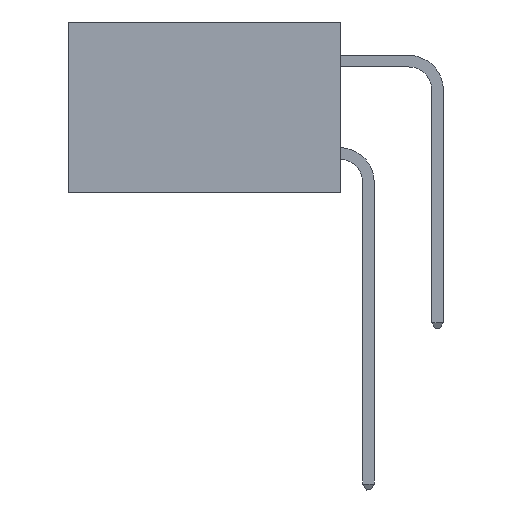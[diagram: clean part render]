
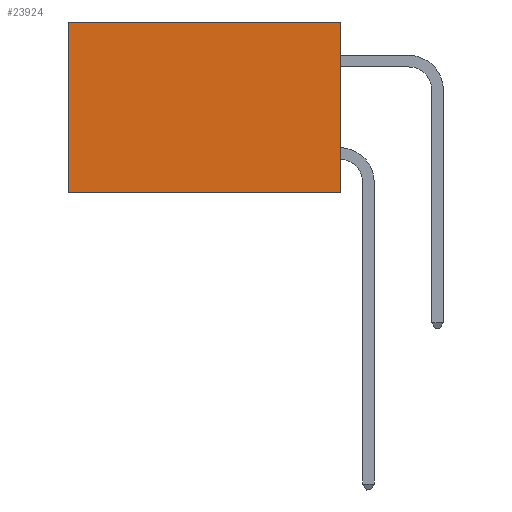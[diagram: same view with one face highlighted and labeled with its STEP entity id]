
A CAD part, left-side view. The second image highlights one B-rep face of the part: STEP entity #23924.
In plain terms, the highlighted planar face has unit normal (-1, 0, 0).
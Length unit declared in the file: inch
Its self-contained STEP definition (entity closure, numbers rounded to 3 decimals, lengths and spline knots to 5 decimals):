
#309 = VERTEX_POINT ( 'NONE', #7056 ) ;
#2380 = PLANE ( 'NONE',  #12014 ) ;
#3453 = VECTOR ( 'NONE', #6082, 39.37008 ) ;
#5882 = VECTOR ( 'NONE', #22699, 39.37008 ) ;
#6082 = DIRECTION ( 'NONE',  ( 0., 0., -1. ) ) ;
#7008 = CARTESIAN_POINT ( 'NONE',  ( 0.277, 0.59, -0.37 ) ) ;
#7056 = CARTESIAN_POINT ( 'NONE',  ( 0.277, 0.59, 0. ) ) ;
#7470 = LINE ( 'NONE', #18677, #13592 ) ;
#7644 = VERTEX_POINT ( 'NONE', #24362 ) ;
#7738 = ORIENTED_EDGE ( 'NONE', *, *, #19756, .T. ) ;
#8578 = CARTESIAN_POINT ( 'NONE',  ( 0.277, 0., 0. ) ) ;
#8808 = CARTESIAN_POINT ( 'NONE',  ( 0.277, 0., -0.37 ) ) ;
#9830 = ORIENTED_EDGE ( 'NONE', *, *, #13328, .T. ) ;
#10345 = LINE ( 'NONE', #26241, #3453 ) ;
#10937 = DIRECTION ( 'NONE',  ( 0., 0., -1. ) ) ;
#11738 = CARTESIAN_POINT ( 'NONE',  ( 0.277, 0., -0.37 ) ) ;
#12014 = AXIS2_PLACEMENT_3D ( 'NONE', #8808, #22921, #10937 ) ;
#12280 = ORIENTED_EDGE ( 'NONE', *, *, #18109, .F. ) ;
#12651 = ORIENTED_EDGE ( 'NONE', *, *, #14563, .F. ) ;
#13328 = EDGE_CURVE ( 'NONE', #7644, #309, #21470, .T. ) ;
#13578 = VERTEX_POINT ( 'NONE', #7008 ) ;
#13592 = VECTOR ( 'NONE', #20657, 39.37008 ) ;
#13837 = DIRECTION ( 'NONE',  ( 0., 1., 0. ) ) ;
#14563 = EDGE_CURVE ( 'NONE', #7644, #19692, #7470, .T. ) ;
#14714 = LINE ( 'NONE', #11738, #24664 ) ;
#17398 = FACE_OUTER_BOUND ( 'NONE', #26008, .T. ) ;
#18109 = EDGE_CURVE ( 'NONE', #19692, #13578, #14714, .T. ) ;
#18677 = CARTESIAN_POINT ( 'NONE',  ( 0.277, 0., -0.37 ) ) ;
#19692 = VERTEX_POINT ( 'NONE', #20237 ) ;
#19756 = EDGE_CURVE ( 'NONE', #309, #13578, #10345, .T. ) ;
#20237 = CARTESIAN_POINT ( 'NONE',  ( 0.277, 0., -0.37 ) ) ;
#20657 = DIRECTION ( 'NONE',  ( 0., 0., -1. ) ) ;
#21470 = LINE ( 'NONE', #8578, #5882 ) ;
#22699 = DIRECTION ( 'NONE',  ( 0., 1., 0. ) ) ;
#22921 = DIRECTION ( 'NONE',  ( 1., 0., 0. ) ) ;
#23924 = ADVANCED_FACE ( 'NONE', ( #17398 ), #2380, .F. ) ;
#24362 = CARTESIAN_POINT ( 'NONE',  ( 0.277, 0., 0. ) ) ;
#24664 = VECTOR ( 'NONE', #13837, 39.37008 ) ;
#26008 = EDGE_LOOP ( 'NONE', ( #7738, #12280, #12651, #9830 ) ) ;
#26241 = CARTESIAN_POINT ( 'NONE',  ( 0.277, 0.59, -0.37 ) ) ;
